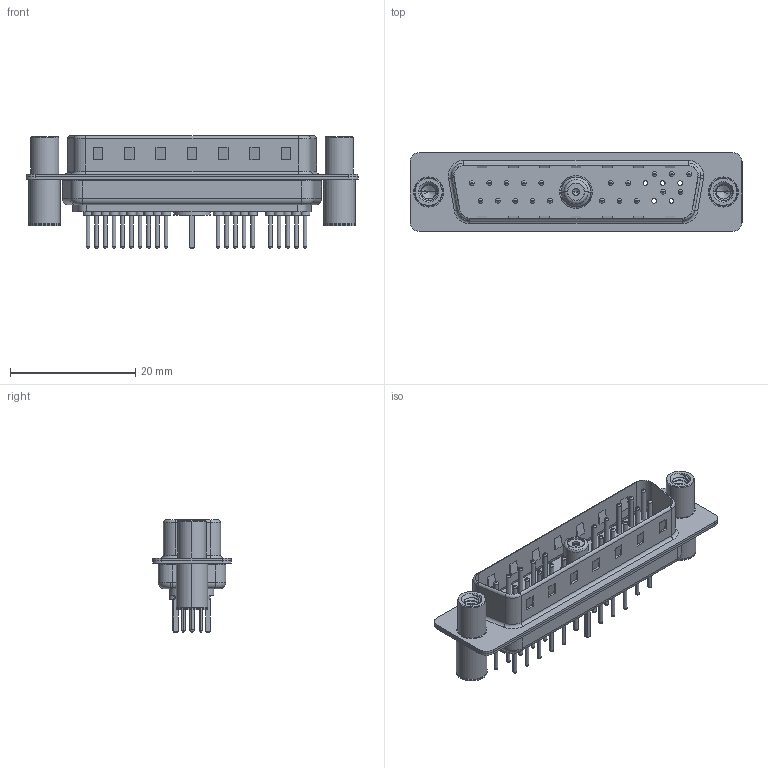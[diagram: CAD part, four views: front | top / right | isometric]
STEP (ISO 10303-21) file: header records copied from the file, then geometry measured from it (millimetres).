
FILE_DESCRIPTION (( 'STEP AP203' ), '1' );
FILE_NAME ('627-21W1624-5N4.STEP', '2019-05-28T02:21:42', ( '' ), ( '' ), 'SwSTEP 2.0', 'SolidWorks 2016', '' );
FILE_SCHEMA (( 'CONFIG_CONTROL_DESIGN' ));
Length unit declared in the file: millimetre
Products named in the file (13): Co-Ax Jack_Straight PC Tail; Locking Collar; 627Combo Contact Row 1_24; Insulator Socket; 627Combo Shell Front_25 Contacts; Insulator Socket 2; 627Combo Housing_21W1; 627Combo Contact Row 2_24; 627-21W1624-5N4; Co-Ax Jack Assy_S; 627Combo Threaded Standoff and Board Spacer_4; 627Combo Shell Rear_25 Contacts; Socket_Str
Assembly tree (31 placements, depth 3):
  627-21W1624-5N4
    627Combo Housing_21W1
    627Combo Shell Rear_25 Contacts
    627Combo Shell Front_25 Contacts
    627Combo Threaded Standoff and Board Spacer_4  x2
    Co-Ax Jack Assy_S
      Co-Ax Jack_Straight PC Tail
      Insulator Socket
      Insulator Socket 2
      Locking Collar
      Socket_Str
    627Combo Contact Row 1_24  x10
    627Combo Contact Row 2_24  x10
Bounding box: 53 x 12.6 x 17.9 mm (x, y, z)
Volume: 3027.3 mm3; surface area: 7761.4 mm2
Topology: 30 solids, 30 shells, 1313 faces, 2912 edges, 1776 vertices
Faces by surface type: cylinder 516, torus 378, plane 364, cone 39, bspline 14, sphere 2
Entity records: 24991 total; most frequent: CARTESIAN_POINT 5927, DIRECTION 3835, ORIENTED_EDGE 3400, EDGE_CURVE 1700, AXIS2_PLACEMENT_3D 1505, VERTEX_POINT 1079, EDGE_LOOP 875, VECTOR 825
